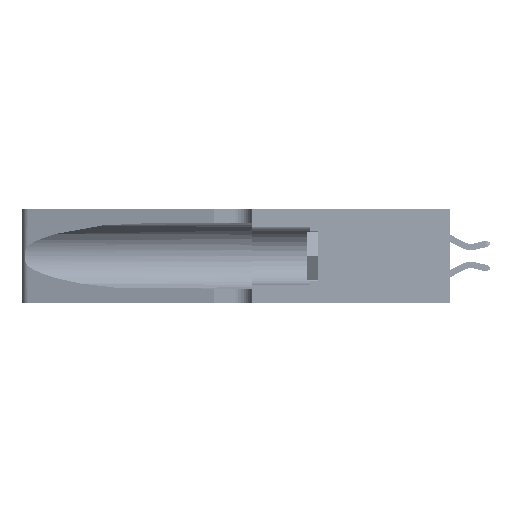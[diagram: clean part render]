
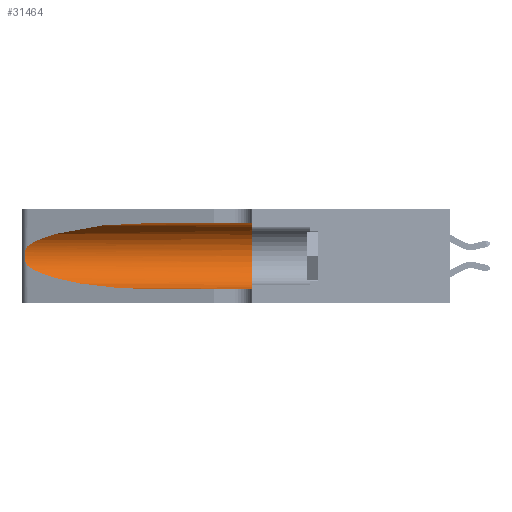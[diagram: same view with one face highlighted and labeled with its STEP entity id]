
A CAD part, left-side view. The second image highlights one B-rep face of the part: STEP entity #31464.
In plain terms, the highlighted cylindrical face has radius 3.308 mm (diameter 6.617 mm), a partial arc.
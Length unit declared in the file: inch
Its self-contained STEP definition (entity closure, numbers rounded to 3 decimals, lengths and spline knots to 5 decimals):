
#32 = CARTESIAN_POINT ( 'NONE',  ( 0.25487, 1.22718, 0.14631 ) ) ;
#858 = EDGE_LOOP ( 'NONE', ( #22228, #28670, #32189, #38819, #11604, #34465 ) ) ;
#947 = CARTESIAN_POINT ( 'NONE',  ( 0.1305, 1.61858, 0.31525 ) ) ;
#2383 = CARTESIAN_POINT ( 'NONE',  ( 0.26018, 1.23835, 0.19895 ) ) ;
#3401 = CARTESIAN_POINT ( 'NONE',  ( 0.18966, 0.96281, 0.31525 ) ) ;
#6030 = CARTESIAN_POINT ( 'NONE',  ( 0.26075, 1.23896, 0.178 ) ) ;
#7050 = CARTESIAN_POINT ( 'NONE',  ( 0.2373, 1.15595, 0.28018 ) ) ;
#7721 = DIRECTION ( 'NONE',  ( 0., -1., 0. ) ) ;
#9607 = CARTESIAN_POINT ( 'NONE',  ( 0.25856, 1.23593, 0.16098 ) ) ;
#9723 = CARTESIAN_POINT ( 'NONE',  ( 0.18966, 0.96281, 0.05475 ) ) ;
#9835 = VECTOR ( 'NONE', #27926, 39.37008 ) ;
#9986 = EDGE_CURVE ( 'NONE', #12784, #17534, #24250, .T. ) ;
#11604 = ORIENTED_EDGE ( 'NONE', *, *, #35420, .F. ) ;
#12784 = VERTEX_POINT ( 'NONE', #32 ) ;
#13010 = CARTESIAN_POINT ( 'NONE',  ( 0.25555, 1.22994, 0.2215 ) ) ;
#13160 = CARTESIAN_POINT ( 'NONE',  ( 0.25639, 1.23186, 0.15144 ) ) ;
#16124 = CYLINDRICAL_SURFACE ( 'NONE', #18341, 0.13025 ) ;
#16723 = CARTESIAN_POINT ( 'NONE',  ( 0.25487, 1.22718, 0.14631 ) ) ;
#16733 = CARTESIAN_POINT ( 'NONE',  ( 0.1305, 0.35, 0.185 ) ) ;
#16763 = CARTESIAN_POINT ( 'NONE',  ( 0.25487, 1.22718, 0.14631 ) ) ;
#17255 = FACE_OUTER_BOUND ( 'NONE', #858, .T. ) ;
#17534 = VERTEX_POINT ( 'NONE', #25991 ) ;
#18341 = AXIS2_PLACEMENT_3D ( 'NONE', #28987, #7721, #32505 ) ;
#18582 = EDGE_CURVE ( 'NONE', #24704, #41707, #34919, .T. ) ;
#19098 = CIRCLE ( 'NONE', #41769, 0.13025 ) ;
#20128 = VERTEX_POINT ( 'NONE', #27042 ) ;
#20161 = CARTESIAN_POINT ( 'NONE',  ( 0.25639, 1.23184, 0.21858 ) ) ;
#20291 = DIRECTION ( 'NONE',  ( 0., 0., 1. ) ) ;
#20397 = LINE ( 'NONE', #42049, #9835 ) ;
#20941 = EDGE_CURVE ( 'NONE', #17534, #32662, #20397, .T. ) ;
#22228 = ORIENTED_EDGE ( 'NONE', *, *, #42211, .T. ) ;
#23723 = CARTESIAN_POINT ( 'NONE',  ( 0.25854, 1.2359, 0.20912 ) ) ;
#23997 = B_SPLINE_CURVE_WITH_KNOTS ( 'NONE', 3,
 ( #37750, #13010, #20161, #44774, #23723, #2383, #27305, #6030, #30847, #9607, #34356, #13160, #37899, #16763 ),
 .UNSPECIFIED., .F., .F.,
 ( 4, 2, 2, 2, 2, 2, 4 ),
 ( 0., 0.00027, 0.00053, 0.00107, 0.0016, 0.00187, 0.00214 ),
 .UNSPECIFIED. ) ;
#24250 =( BOUNDED_CURVE ( )  B_SPLINE_CURVE ( 3, ( #16723, #30967, #9723, #34478 ),
 .UNSPECIFIED., .F., .T. ) 
 B_SPLINE_CURVE_WITH_KNOTS ( ( 4, 4 ),
 ( 3.44316, 4.71239 ),
 .UNSPECIFIED. ) 
 CURVE ( )  GEOMETRIC_REPRESENTATION_ITEM ( )  RATIONAL_B_SPLINE_CURVE ( ( 1., 0.87, 0.87, 1. ) ) 
 REPRESENTATION_ITEM ( '' )  );
#24695 = CARTESIAN_POINT ( 'NONE',  ( 0.1305, 0.72297, 0.31525 ) ) ;
#24704 = VERTEX_POINT ( 'NONE', #40086 ) ;
#25912 = DIRECTION ( 'NONE',  ( 0., -1., 0. ) ) ;
#25991 = CARTESIAN_POINT ( 'NONE',  ( 0.1305, 0.72297, 0.05475 ) ) ;
#27042 = CARTESIAN_POINT ( 'NONE',  ( 0.25487, 1.22718, 0.22369 ) ) ;
#27305 = CARTESIAN_POINT ( 'NONE',  ( 0.26075, 1.23896, 0.19203 ) ) ;
#27926 = DIRECTION ( 'NONE',  ( 0., -1., 0. ) ) ;
#28102 = CARTESIAN_POINT ( 'NONE',  ( 0.1305, 0.35, 0.05475 ) ) ;
#28670 = ORIENTED_EDGE ( 'NONE', *, *, #43069, .T. ) ;
#28987 = CARTESIAN_POINT ( 'NONE',  ( 0.1305, 1.61858, 0.185 ) ) ;
#29116 = CARTESIAN_POINT ( 'NONE',  ( 0.1305, 0.35, 0.31525 ) ) ;
#30847 = CARTESIAN_POINT ( 'NONE',  ( 0.26017, 1.23833, 0.17102 ) ) ;
#30967 = CARTESIAN_POINT ( 'NONE',  ( 0.2373, 1.15595, 0.08982 ) ) ;
#31464 = ADVANCED_FACE ( 'NONE', ( #17255 ), #16124, .F. ) ;
#31838 = CARTESIAN_POINT ( 'NONE',  ( 0.25487, 1.22718, 0.22369 ) ) ;
#32189 = ORIENTED_EDGE ( 'NONE', *, *, #9986, .T. ) ;
#32505 = DIRECTION ( 'NONE',  ( 0., 0., -1. ) ) ;
#32662 = VERTEX_POINT ( 'NONE', #28102 ) ;
#34356 = CARTESIAN_POINT ( 'NONE',  ( 0.25789, 1.23486, 0.15765 ) ) ;
#34465 = ORIENTED_EDGE ( 'NONE', *, *, #18582, .F. ) ;
#34478 = CARTESIAN_POINT ( 'NONE',  ( 0.1305, 0.72297, 0.05475 ) ) ;
#34919 = LINE ( 'NONE', #947, #36028 ) ;
#35420 = EDGE_CURVE ( 'NONE', #41707, #32662, #19098, .T. ) ;
#36028 = VECTOR ( 'NONE', #25912, 39.37008 ) ;
#37750 = CARTESIAN_POINT ( 'NONE',  ( 0.25487, 1.22718, 0.22369 ) ) ;
#37899 = CARTESIAN_POINT ( 'NONE',  ( 0.25555, 1.22993, 0.14849 ) ) ;
#38819 = ORIENTED_EDGE ( 'NONE', *, *, #20941, .T. ) ;
#40086 = CARTESIAN_POINT ( 'NONE',  ( 0.1305, 0.72297, 0.31525 ) ) ;
#41416 = DIRECTION ( 'NONE',  ( 0., 1., 0. ) ) ;
#41707 = VERTEX_POINT ( 'NONE', #29116 ) ;
#41769 = AXIS2_PLACEMENT_3D ( 'NONE', #16733, #41416, #20291 ) ;
#42049 = CARTESIAN_POINT ( 'NONE',  ( 0.1305, 1.61858, 0.05475 ) ) ;
#42211 = EDGE_CURVE ( 'NONE', #24704, #20128, #45370, .T. ) ;
#43069 = EDGE_CURVE ( 'NONE', #20128, #12784, #23997, .T. ) ;
#44774 = CARTESIAN_POINT ( 'NONE',  ( 0.25787, 1.23484, 0.2124 ) ) ;
#45370 =( BOUNDED_CURVE ( )  B_SPLINE_CURVE ( 3, ( #24695, #3401, #7050, #31838 ),
 .UNSPECIFIED., .F., .F. ) 
 B_SPLINE_CURVE_WITH_KNOTS ( ( 4, 4 ),
 ( 1.5708, 2.84003 ),
 .UNSPECIFIED. ) 
 CURVE ( )  GEOMETRIC_REPRESENTATION_ITEM ( )  RATIONAL_B_SPLINE_CURVE ( ( 1., 0.87, 0.87, 1. ) ) 
 REPRESENTATION_ITEM ( '' )  );
